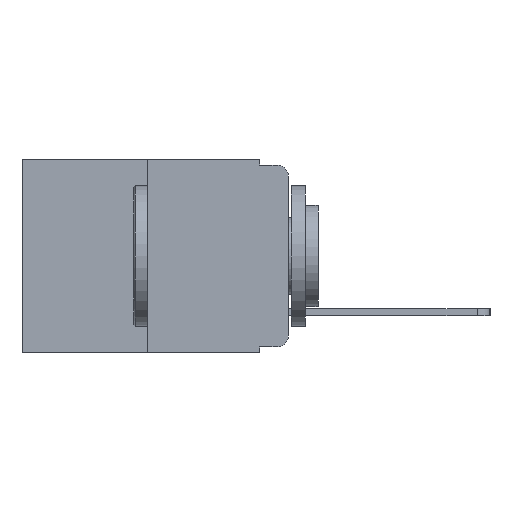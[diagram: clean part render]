
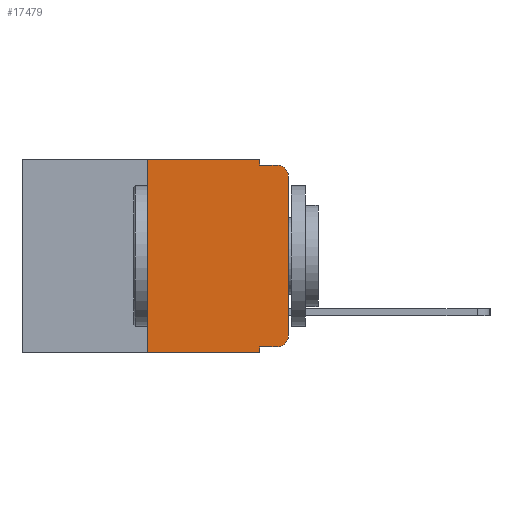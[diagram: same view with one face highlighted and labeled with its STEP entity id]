
A CAD part, left-side view. The second image highlights one B-rep face of the part: STEP entity #17479.
In plain terms, the highlighted planar face has unit normal (-1, 0, 0).
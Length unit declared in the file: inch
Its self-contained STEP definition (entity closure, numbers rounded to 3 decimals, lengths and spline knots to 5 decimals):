
#94 = LINE ( 'NONE', #17475, #13939 ) ;
#272 = ORIENTED_EDGE ( 'NONE', *, *, #13259, .F. ) ;
#385 = CARTESIAN_POINT ( 'NONE',  ( 0., 0.051, 0. ) ) ;
#499 = ORIENTED_EDGE ( 'NONE', *, *, #9838, .T. ) ;
#711 = ORIENTED_EDGE ( 'NONE', *, *, #16676, .T. ) ;
#804 = ORIENTED_EDGE ( 'NONE', *, *, #15525, .F. ) ;
#928 = EDGE_CURVE ( 'NONE', #7020, #21786, #94, .T. ) ;
#1073 = VECTOR ( 'NONE', #10369, 39.37008 ) ;
#1149 = ORIENTED_EDGE ( 'NONE', *, *, #22252, .T. ) ;
#1188 = LINE ( 'NONE', #8507, #10334 ) ;
#1606 = CARTESIAN_POINT ( 'NONE',  ( 0., 0.02, -0.313 ) ) ;
#1777 = VERTEX_POINT ( 'NONE', #10914 ) ;
#1831 = DIRECTION ( 'NONE',  ( 0., 0., 1. ) ) ;
#2601 = VECTOR ( 'NONE', #1831, 39.37008 ) ;
#3251 = VERTEX_POINT ( 'NONE', #6729 ) ;
#3287 = FACE_OUTER_BOUND ( 'NONE', #13146, .T. ) ;
#3591 = DIRECTION ( 'NONE',  ( 0., 0., -1. ) ) ;
#3818 = CARTESIAN_POINT ( 'NONE',  ( 0., 0.051, 0. ) ) ;
#4011 = CIRCLE ( 'NONE', #10051, 0.02 ) ;
#4284 = ORIENTED_EDGE ( 'NONE', *, *, #10973, .F. ) ;
#4468 = LINE ( 'NONE', #3818, #8659 ) ;
#5007 = ORIENTED_EDGE ( 'NONE', *, *, #14413, .F. ) ;
#5544 = ORIENTED_EDGE ( 'NONE', *, *, #928, .F. ) ;
#5640 = CARTESIAN_POINT ( 'NONE',  ( 0., 0.051, -0.01 ) ) ;
#5770 = VECTOR ( 'NONE', #16834, 39.37008 ) ;
#6024 = DIRECTION ( 'NONE',  ( 1., 0., 0. ) ) ;
#6307 = VERTEX_POINT ( 'NONE', #15227 ) ;
#6437 = VERTEX_POINT ( 'NONE', #15590 ) ;
#6729 = CARTESIAN_POINT ( 'NONE',  ( 0., 0.051, -0.01 ) ) ;
#6773 = DIRECTION ( 'NONE',  ( 0., -1., 0. ) ) ;
#7020 = VERTEX_POINT ( 'NONE', #12070 ) ;
#7073 = VECTOR ( 'NONE', #11333, 39.37008 ) ;
#7526 = LINE ( 'NONE', #14273, #2601 ) ;
#7584 = AXIS2_PLACEMENT_3D ( 'NONE', #8688, #20598, #10410 ) ;
#7887 = ORIENTED_EDGE ( 'NONE', *, *, #8685, .T. ) ;
#8006 = CIRCLE ( 'NONE', #7584, 0.02 ) ;
#8340 = LINE ( 'NONE', #5640, #11804 ) ;
#8445 = VERTEX_POINT ( 'NONE', #18509 ) ;
#8507 = CARTESIAN_POINT ( 'NONE',  ( 0., 0.051, -0.333 ) ) ;
#8659 = VECTOR ( 'NONE', #15969, 39.37008 ) ;
#8685 = EDGE_CURVE ( 'NONE', #11518, #6437, #4011, .T. ) ;
#8688 = CARTESIAN_POINT ( 'NONE',  ( 0., 0.02, -0.03 ) ) ;
#9491 = PLANE ( 'NONE',  #10898 ) ;
#9838 = EDGE_CURVE ( 'NONE', #19524, #11518, #1188, .T. ) ;
#10051 = AXIS2_PLACEMENT_3D ( 'NONE', #1606, #14073, #3591 ) ;
#10174 = CARTESIAN_POINT ( 'NONE',  ( 0., 0.051, -0.333 ) ) ;
#10334 = VECTOR ( 'NONE', #6773, 39.37008 ) ;
#10369 = DIRECTION ( 'NONE',  ( 0., 0., 1. ) ) ;
#10410 = DIRECTION ( 'NONE',  ( 0., 0., -1. ) ) ;
#10898 = AXIS2_PLACEMENT_3D ( 'NONE', #11125, #6024, #18012 ) ;
#10914 = CARTESIAN_POINT ( 'NONE',  ( 0., 0.02, -0.01 ) ) ;
#10973 = EDGE_CURVE ( 'NONE', #19524, #12721, #20669, .T. ) ;
#11020 = CARTESIAN_POINT ( 'NONE',  ( 0., 0.02, -0.333 ) ) ;
#11125 = CARTESIAN_POINT ( 'NONE',  ( 0., 0.473, 0. ) ) ;
#11333 = DIRECTION ( 'NONE',  ( 0., 0., -1. ) ) ;
#11518 = VERTEX_POINT ( 'NONE', #11020 ) ;
#11804 = VECTOR ( 'NONE', #19381, 39.37008 ) ;
#12070 = CARTESIAN_POINT ( 'NONE',  ( 0., 0.25, 0. ) ) ;
#12721 = VERTEX_POINT ( 'NONE', #17528 ) ;
#13146 = EDGE_LOOP ( 'NONE', ( #20007, #711, #804, #5007, #5544, #272, #1149, #4284, #499, #7887 ) ) ;
#13259 = EDGE_CURVE ( 'NONE', #6307, #7020, #7526, .T. ) ;
#13939 = VECTOR ( 'NONE', #20541, 39.37008 ) ;
#14073 = DIRECTION ( 'NONE',  ( -1., 0., 0. ) ) ;
#14273 = CARTESIAN_POINT ( 'NONE',  ( 0., 0.25, 0. ) ) ;
#14413 = EDGE_CURVE ( 'NONE', #21786, #3251, #4468, .T. ) ;
#15140 = CARTESIAN_POINT ( 'NONE',  ( 0., 0.473, -0.343 ) ) ;
#15227 = CARTESIAN_POINT ( 'NONE',  ( 0., 0.25, -0.343 ) ) ;
#15525 = EDGE_CURVE ( 'NONE', #3251, #1777, #8340, .T. ) ;
#15590 = CARTESIAN_POINT ( 'NONE',  ( 0., 0., -0.313 ) ) ;
#15969 = DIRECTION ( 'NONE',  ( 0., 0., -1. ) ) ;
#16676 = EDGE_CURVE ( 'NONE', #8445, #1777, #8006, .T. ) ;
#16834 = DIRECTION ( 'NONE',  ( 0., -1., 0. ) ) ;
#17475 = CARTESIAN_POINT ( 'NONE',  ( 0., 0.473, 0. ) ) ;
#17479 = ADVANCED_FACE ( 'NONE', ( #3287 ), #9491, .F. ) ;
#17528 = CARTESIAN_POINT ( 'NONE',  ( 0., 0.051, -0.343 ) ) ;
#17795 = EDGE_CURVE ( 'NONE', #6437, #8445, #18733, .T. ) ;
#18012 = DIRECTION ( 'NONE',  ( 0., 0., -1. ) ) ;
#18509 = CARTESIAN_POINT ( 'NONE',  ( 0., 0., -0.03 ) ) ;
#18733 = LINE ( 'NONE', #22264, #1073 ) ;
#19006 = CARTESIAN_POINT ( 'NONE',  ( 0., 0.051, 0. ) ) ;
#19381 = DIRECTION ( 'NONE',  ( 0., -1., 0. ) ) ;
#19466 = LINE ( 'NONE', #15140, #5770 ) ;
#19524 = VERTEX_POINT ( 'NONE', #10174 ) ;
#20007 = ORIENTED_EDGE ( 'NONE', *, *, #17795, .T. ) ;
#20541 = DIRECTION ( 'NONE',  ( 0., -1., 0. ) ) ;
#20598 = DIRECTION ( 'NONE',  ( -1., 0., 0. ) ) ;
#20669 = LINE ( 'NONE', #385, #7073 ) ;
#21786 = VERTEX_POINT ( 'NONE', #19006 ) ;
#22252 = EDGE_CURVE ( 'NONE', #6307, #12721, #19466, .T. ) ;
#22264 = CARTESIAN_POINT ( 'NONE',  ( 0., 0., 0. ) ) ;
